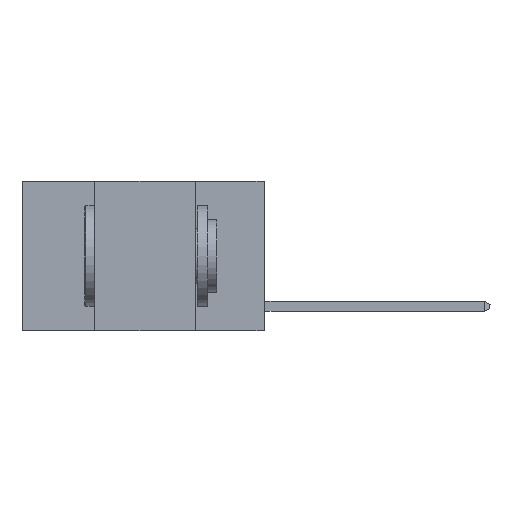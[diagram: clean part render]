
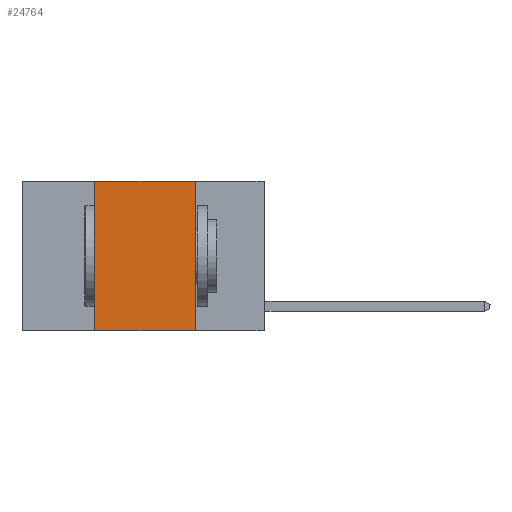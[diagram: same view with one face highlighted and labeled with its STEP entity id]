
A CAD part, left-side view. The second image highlights one B-rep face of the part: STEP entity #24764.
In plain terms, the highlighted planar face has unit normal (-1, 0, 0).
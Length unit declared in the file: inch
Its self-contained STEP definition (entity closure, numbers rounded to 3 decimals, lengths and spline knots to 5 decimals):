
#375 = CARTESIAN_POINT ( 'NONE',  ( 0., 0.17, 0. ) ) ;
#1116 = VECTOR ( 'NONE', #9462, 39.37008 ) ;
#2610 = CARTESIAN_POINT ( 'NONE',  ( 0., 0.42, 0. ) ) ;
#3280 = LINE ( 'NONE', #27289, #7975 ) ;
#3365 = CARTESIAN_POINT ( 'NONE',  ( 0., 0.6, 0. ) ) ;
#3867 = VERTEX_POINT ( 'NONE', #23705 ) ;
#4394 = LINE ( 'NONE', #28540, #11571 ) ;
#5687 = EDGE_LOOP ( 'NONE', ( #12660, #7416, #27207, #26317 ) ) ;
#6387 = EDGE_CURVE ( 'NONE', #7877, #3867, #4394, .T. ) ;
#6942 = DIRECTION ( 'NONE',  ( 0., 0., -1. ) ) ;
#7002 = EDGE_CURVE ( 'NONE', #18478, #7877, #3280, .T. ) ;
#7268 = EDGE_CURVE ( 'NONE', #30530, #18478, #28512, .T. ) ;
#7416 = ORIENTED_EDGE ( 'NONE', *, *, #7002, .F. ) ;
#7449 = AXIS2_PLACEMENT_3D ( 'NONE', #3365, #24713, #30025 ) ;
#7877 = VERTEX_POINT ( 'NONE', #375 ) ;
#7975 = VECTOR ( 'NONE', #24931, 39.37008 ) ;
#9093 = DIRECTION ( 'NONE',  ( 0., -1., 0. ) ) ;
#9462 = DIRECTION ( 'NONE',  ( 0., 0., 1. ) ) ;
#10429 = VECTOR ( 'NONE', #9093, 39.37008 ) ;
#10501 = EDGE_CURVE ( 'NONE', #30530, #3867, #11457, .T. ) ;
#11457 = LINE ( 'NONE', #21091, #10429 ) ;
#11571 = VECTOR ( 'NONE', #6942, 39.37008 ) ;
#12660 = ORIENTED_EDGE ( 'NONE', *, *, #6387, .F. ) ;
#15431 = PLANE ( 'NONE',  #7449 ) ;
#16532 = CARTESIAN_POINT ( 'NONE',  ( 0., 0.42, -0.37 ) ) ;
#18478 = VERTEX_POINT ( 'NONE', #2610 ) ;
#21091 = CARTESIAN_POINT ( 'NONE',  ( 0., 0.6, -0.37 ) ) ;
#23705 = CARTESIAN_POINT ( 'NONE',  ( 0., 0.17, -0.37 ) ) ;
#24713 = DIRECTION ( 'NONE',  ( 1., 0., 0. ) ) ;
#24764 = ADVANCED_FACE ( 'NONE', ( #27055 ), #15431, .F. ) ;
#24931 = DIRECTION ( 'NONE',  ( 0., -1., 0. ) ) ;
#26317 = ORIENTED_EDGE ( 'NONE', *, *, #10501, .T. ) ;
#27055 = FACE_OUTER_BOUND ( 'NONE', #5687, .T. ) ;
#27207 = ORIENTED_EDGE ( 'NONE', *, *, #7268, .F. ) ;
#27289 = CARTESIAN_POINT ( 'NONE',  ( 0., 0.6, 0. ) ) ;
#28512 = LINE ( 'NONE', #28987, #1116 ) ;
#28540 = CARTESIAN_POINT ( 'NONE',  ( 0., 0.17, 0. ) ) ;
#28987 = CARTESIAN_POINT ( 'NONE',  ( 0., 0.42, 0. ) ) ;
#30025 = DIRECTION ( 'NONE',  ( 0., 0., -1. ) ) ;
#30530 = VERTEX_POINT ( 'NONE', #16532 ) ;
